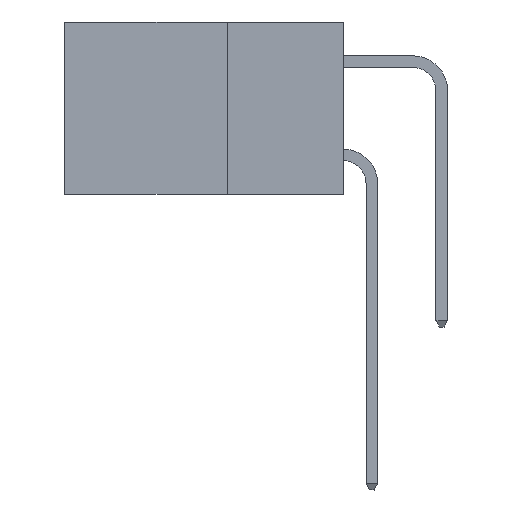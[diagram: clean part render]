
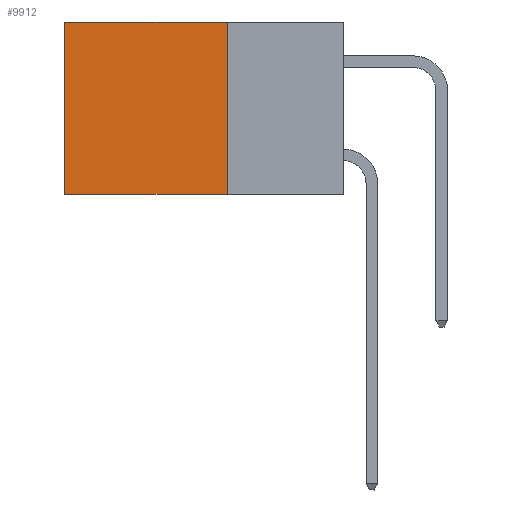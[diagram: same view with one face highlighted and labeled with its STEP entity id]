
A CAD part, left-side view. The second image highlights one B-rep face of the part: STEP entity #9912.
In plain terms, the highlighted planar face has unit normal (-1, 0, 0).
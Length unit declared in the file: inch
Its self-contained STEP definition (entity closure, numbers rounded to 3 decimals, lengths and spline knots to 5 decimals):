
#92 = CARTESIAN_POINT ( 'NONE',  ( 0.2615, 0.25, -0.37 ) ) ;
#1284 = ORIENTED_EDGE ( 'NONE', *, *, #5863, .F. ) ;
#1869 = AXIS2_PLACEMENT_3D ( 'NONE', #19400, #10384, #13640 ) ;
#3166 = FACE_OUTER_BOUND ( 'NONE', #6554, .T. ) ;
#3276 = VECTOR ( 'NONE', #15694, 39.37008 ) ;
#3656 = DIRECTION ( 'NONE',  ( 0., 1., 0. ) ) ;
#3746 = LINE ( 'NONE', #92, #8453 ) ;
#4066 = ORIENTED_EDGE ( 'NONE', *, *, #10737, .T. ) ;
#4250 = EDGE_CURVE ( 'NONE', #9289, #7118, #15893, .T. ) ;
#4823 = DIRECTION ( 'NONE',  ( 0., 0., -1. ) ) ;
#5863 = EDGE_CURVE ( 'NONE', #6606, #14265, #6214, .T. ) ;
#6214 = LINE ( 'NONE', #9565, #13451 ) ;
#6373 = CARTESIAN_POINT ( 'NONE',  ( 0.2615, 0.25, -0.37 ) ) ;
#6491 = VECTOR ( 'NONE', #17679, 39.37008 ) ;
#6554 = EDGE_LOOP ( 'NONE', ( #7303, #12051, #1284, #4066 ) ) ;
#6606 = VERTEX_POINT ( 'NONE', #9461 ) ;
#7055 = CARTESIAN_POINT ( 'NONE',  ( 0.2615, 0.6, 0. ) ) ;
#7118 = VERTEX_POINT ( 'NONE', #15565 ) ;
#7303 = ORIENTED_EDGE ( 'NONE', *, *, #4250, .T. ) ;
#8453 = VECTOR ( 'NONE', #3656, 39.37008 ) ;
#8887 = PLANE ( 'NONE',  #1869 ) ;
#9289 = VERTEX_POINT ( 'NONE', #7055 ) ;
#9461 = CARTESIAN_POINT ( 'NONE',  ( 0.2615, 0.25, 0. ) ) ;
#9565 = CARTESIAN_POINT ( 'NONE',  ( 0.2615, 0.25, -0.37 ) ) ;
#9912 = ADVANCED_FACE ( 'NONE', ( #3166 ), #8887, .F. ) ;
#10384 = DIRECTION ( 'NONE',  ( 1., 0., 0. ) ) ;
#10737 = EDGE_CURVE ( 'NONE', #6606, #9289, #12806, .T. ) ;
#11321 = CARTESIAN_POINT ( 'NONE',  ( 0.2615, 0.25, 0. ) ) ;
#12051 = ORIENTED_EDGE ( 'NONE', *, *, #15494, .F. ) ;
#12806 = LINE ( 'NONE', #11321, #3276 ) ;
#13302 = CARTESIAN_POINT ( 'NONE',  ( 0.2615, 0.6, -0.37 ) ) ;
#13451 = VECTOR ( 'NONE', #4823, 39.37008 ) ;
#13640 = DIRECTION ( 'NONE',  ( 0., 0., -1. ) ) ;
#14265 = VERTEX_POINT ( 'NONE', #6373 ) ;
#15494 = EDGE_CURVE ( 'NONE', #14265, #7118, #3746, .T. ) ;
#15565 = CARTESIAN_POINT ( 'NONE',  ( 0.2615, 0.6, -0.37 ) ) ;
#15694 = DIRECTION ( 'NONE',  ( 0., 1., 0. ) ) ;
#15893 = LINE ( 'NONE', #13302, #6491 ) ;
#17679 = DIRECTION ( 'NONE',  ( 0., 0., -1. ) ) ;
#19400 = CARTESIAN_POINT ( 'NONE',  ( 0.2615, 0.25, -0.37 ) ) ;
